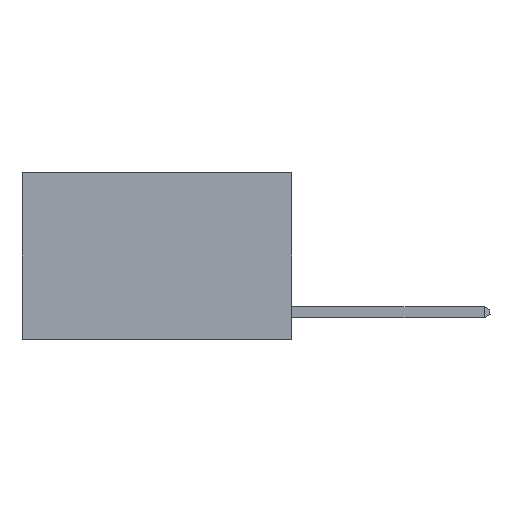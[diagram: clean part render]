
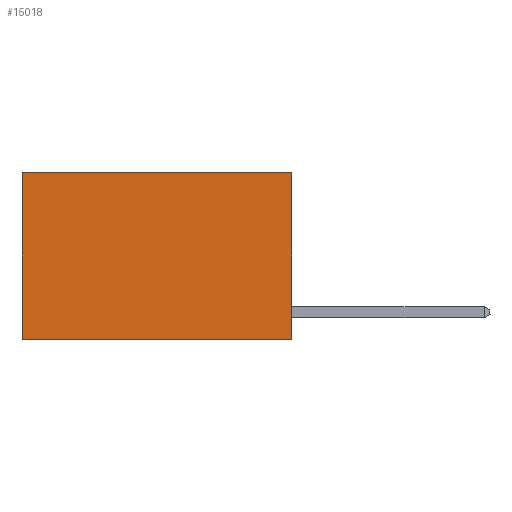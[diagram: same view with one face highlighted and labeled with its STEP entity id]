
A CAD part, left-side view. The second image highlights one B-rep face of the part: STEP entity #15018.
In plain terms, the highlighted planar face has unit normal (-1, 0, 0).
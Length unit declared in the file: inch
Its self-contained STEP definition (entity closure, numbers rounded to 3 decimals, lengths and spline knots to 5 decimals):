
#114 = FACE_OUTER_BOUND ( 'NONE', #5187, .T. ) ;
#422 = CARTESIAN_POINT ( 'NONE',  ( 0.2625, 0.6, 0. ) ) ;
#599 = DIRECTION ( 'NONE',  ( 0., 0., -1. ) ) ;
#1679 = DIRECTION ( 'NONE',  ( 0., 0., -1. ) ) ;
#1787 = ORIENTED_EDGE ( 'NONE', *, *, #14461, .F. ) ;
#3347 = VECTOR ( 'NONE', #4978, 39.37008 ) ;
#3435 = ORIENTED_EDGE ( 'NONE', *, *, #4547, .T. ) ;
#3922 = VERTEX_POINT ( 'NONE', #17666 ) ;
#4547 = EDGE_CURVE ( 'NONE', #14622, #13436, #15597, .T. ) ;
#4978 = DIRECTION ( 'NONE',  ( 0., 0., -1. ) ) ;
#5158 = LINE ( 'NONE', #18385, #3347 ) ;
#5185 = CARTESIAN_POINT ( 'NONE',  ( 0.2625, 0., 0. ) ) ;
#5187 = EDGE_LOOP ( 'NONE', ( #3435, #1787, #7809, #13947 ) ) ;
#5588 = LINE ( 'NONE', #10099, #15579 ) ;
#6151 = PLANE ( 'NONE',  #14644 ) ;
#7161 = EDGE_CURVE ( 'NONE', #11277, #14622, #19152, .T. ) ;
#7809 = ORIENTED_EDGE ( 'NONE', *, *, #13448, .F. ) ;
#8574 = VECTOR ( 'NONE', #17573, 39.37008 ) ;
#9199 = CARTESIAN_POINT ( 'NONE',  ( 0.2625, 0., 0. ) ) ;
#10060 = CARTESIAN_POINT ( 'NONE',  ( 0.2625, 0., 0. ) ) ;
#10099 = CARTESIAN_POINT ( 'NONE',  ( 0.2625, 0., -0.37 ) ) ;
#10770 = CARTESIAN_POINT ( 'NONE',  ( 0.2625, 0.6, -0.37 ) ) ;
#10938 = CARTESIAN_POINT ( 'NONE',  ( 0.2625, 0.6, 0. ) ) ;
#11277 = VERTEX_POINT ( 'NONE', #5185 ) ;
#13436 = VERTEX_POINT ( 'NONE', #10770 ) ;
#13448 = EDGE_CURVE ( 'NONE', #11277, #3922, #5158, .T. ) ;
#13947 = ORIENTED_EDGE ( 'NONE', *, *, #7161, .T. ) ;
#14461 = EDGE_CURVE ( 'NONE', #3922, #13436, #5588, .T. ) ;
#14622 = VERTEX_POINT ( 'NONE', #422 ) ;
#14644 = AXIS2_PLACEMENT_3D ( 'NONE', #9199, #15228, #599 ) ;
#15018 = ADVANCED_FACE ( 'NONE', ( #114 ), #6151, .F. ) ;
#15228 = DIRECTION ( 'NONE',  ( 1., 0., 0. ) ) ;
#15579 = VECTOR ( 'NONE', #16134, 39.37008 ) ;
#15597 = LINE ( 'NONE', #10938, #17957 ) ;
#16134 = DIRECTION ( 'NONE',  ( 0., 1., 0. ) ) ;
#17573 = DIRECTION ( 'NONE',  ( 0., 1., 0. ) ) ;
#17666 = CARTESIAN_POINT ( 'NONE',  ( 0.2625, 0., -0.37 ) ) ;
#17957 = VECTOR ( 'NONE', #1679, 39.37008 ) ;
#18385 = CARTESIAN_POINT ( 'NONE',  ( 0.2625, 0., 0. ) ) ;
#19152 = LINE ( 'NONE', #10060, #8574 ) ;
